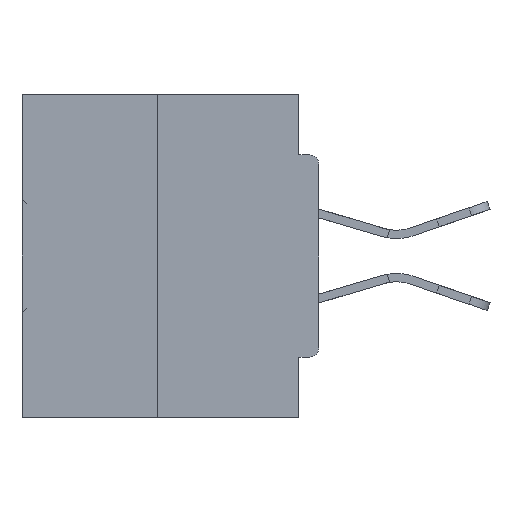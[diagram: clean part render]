
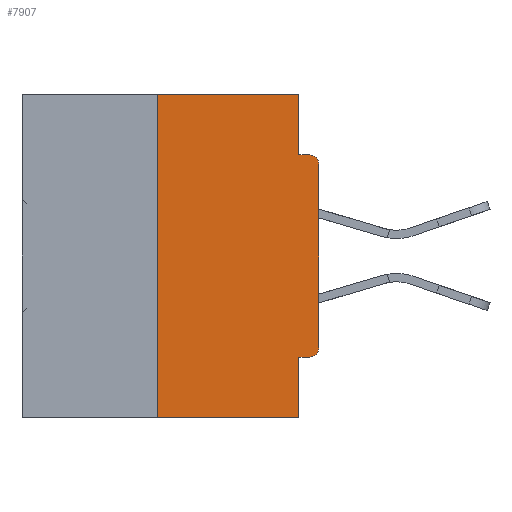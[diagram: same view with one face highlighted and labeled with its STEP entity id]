
A CAD part, left-side view. The second image highlights one B-rep face of the part: STEP entity #7907.
In plain terms, the highlighted planar face has unit normal (-1, 0, 0).
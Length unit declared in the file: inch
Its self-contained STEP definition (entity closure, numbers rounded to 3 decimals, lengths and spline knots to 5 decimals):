
#68 = EDGE_CURVE ( 'NONE', #37832, #5173, #34704, .T. ) ;
#842 = AXIS2_PLACEMENT_3D ( 'NONE', #13772, #17522, #3636 ) ;
#2260 = ORIENTED_EDGE ( 'NONE', *, *, #18033, .F. ) ;
#2802 = CIRCLE ( 'NONE', #25393, 0.015 ) ;
#2816 = CARTESIAN_POINT ( 'NONE',  ( 0., 0.46, -0.5 ) ) ;
#3636 = DIRECTION ( 'NONE',  ( 0., 0., -1. ) ) ;
#4621 = ORIENTED_EDGE ( 'NONE', *, *, #36298, .F. ) ;
#5173 = VERTEX_POINT ( 'NONE', #24727 ) ;
#6350 = VERTEX_POINT ( 'NONE', #41463 ) ;
#7907 = ADVANCED_FACE ( 'NONE', ( #33130 ), #37365, .F. ) ;
#7969 = VECTOR ( 'NONE', #12500, 39.37008 ) ;
#8008 = AXIS2_PLACEMENT_3D ( 'NONE', #12619, #29827, #40417 ) ;
#8057 = CARTESIAN_POINT ( 'NONE',  ( 0., 0.015, -0.4065 ) ) ;
#8179 = VERTEX_POINT ( 'NONE', #10963 ) ;
#8391 = CARTESIAN_POINT ( 'NONE',  ( 0., 0.015, -0.3915 ) ) ;
#8862 = EDGE_CURVE ( 'NONE', #6350, #8179, #31970, .T. ) ;
#10740 = ORIENTED_EDGE ( 'NONE', *, *, #24959, .T. ) ;
#10963 = CARTESIAN_POINT ( 'NONE',  ( 0., 0.031, 0. ) ) ;
#12485 = CARTESIAN_POINT ( 'NONE',  ( 0., 0.031, -0.5 ) ) ;
#12500 = DIRECTION ( 'NONE',  ( 0., -1., 0. ) ) ;
#12554 = EDGE_CURVE ( 'NONE', #15372, #35656, #46511, .T. ) ;
#12619 = CARTESIAN_POINT ( 'NONE',  ( 0., 0.46, 0. ) ) ;
#13407 = ORIENTED_EDGE ( 'NONE', *, *, #38456, .T. ) ;
#13772 = CARTESIAN_POINT ( 'NONE',  ( 0., 0.015, -0.1085 ) ) ;
#14256 = CARTESIAN_POINT ( 'NONE',  ( 0., 0.031, -0.5 ) ) ;
#15091 = LINE ( 'NONE', #36311, #45833 ) ;
#15372 = VERTEX_POINT ( 'NONE', #19482 ) ;
#15651 = EDGE_LOOP ( 'NONE', ( #20581, #33286, #10740, #20710, #2260, #42839, #32192, #13407, #17496, #4621 ) ) ;
#17496 = ORIENTED_EDGE ( 'NONE', *, *, #28105, .F. ) ;
#17522 = DIRECTION ( 'NONE',  ( -1., 0., 0. ) ) ;
#18033 = EDGE_CURVE ( 'NONE', #22012, #15372, #15091, .T. ) ;
#19200 = DIRECTION ( 'NONE',  ( 0., 0., -1. ) ) ;
#19482 = CARTESIAN_POINT ( 'NONE',  ( 0., 0.031, -0.4065 ) ) ;
#19900 = VERTEX_POINT ( 'NONE', #40182 ) ;
#20055 = VERTEX_POINT ( 'NONE', #34281 ) ;
#20581 = ORIENTED_EDGE ( 'NONE', *, *, #8862, .F. ) ;
#20710 = ORIENTED_EDGE ( 'NONE', *, *, #12554, .F. ) ;
#22012 = VERTEX_POINT ( 'NONE', #8057 ) ;
#22480 = DIRECTION ( 'NONE',  ( 0., -1., 0. ) ) ;
#23924 = EDGE_CURVE ( 'NONE', #22012, #37832, #2802, .T. ) ;
#24554 = VECTOR ( 'NONE', #38696, 39.37008 ) ;
#24727 = CARTESIAN_POINT ( 'NONE',  ( 0., 0., -0.1085 ) ) ;
#24959 = EDGE_CURVE ( 'NONE', #19900, #35656, #35084, .T. ) ;
#25393 = AXIS2_PLACEMENT_3D ( 'NONE', #8391, #33586, #44413 ) ;
#25559 = CARTESIAN_POINT ( 'NONE',  ( 0., 0.031, -0.0935 ) ) ;
#25653 = CIRCLE ( 'NONE', #842, 0.015 ) ;
#25705 = CARTESIAN_POINT ( 'NONE',  ( 0., 0., -0.3915 ) ) ;
#26030 = CARTESIAN_POINT ( 'NONE',  ( 0., 0., -0.0935 ) ) ;
#26274 = LINE ( 'NONE', #40622, #33050 ) ;
#26951 = CARTESIAN_POINT ( 'NONE',  ( 0., 0., 0. ) ) ;
#27694 = VECTOR ( 'NONE', #31538, 39.37008 ) ;
#28058 = VERTEX_POINT ( 'NONE', #25559 ) ;
#28105 = EDGE_CURVE ( 'NONE', #28058, #20055, #29544, .T. ) ;
#28616 = DIRECTION ( 'NONE',  ( 0., 0., -1. ) ) ;
#29544 = LINE ( 'NONE', #26030, #43735 ) ;
#29827 = DIRECTION ( 'NONE',  ( 1., 0., 0. ) ) ;
#31538 = DIRECTION ( 'NONE',  ( 0., -1., 0. ) ) ;
#31970 = LINE ( 'NONE', #46102, #7969 ) ;
#32184 = EDGE_CURVE ( 'NONE', #19900, #6350, #34268, .T. ) ;
#32192 = ORIENTED_EDGE ( 'NONE', *, *, #68, .T. ) ;
#33050 = VECTOR ( 'NONE', #19200, 39.37008 ) ;
#33130 = FACE_OUTER_BOUND ( 'NONE', #15651, .T. ) ;
#33286 = ORIENTED_EDGE ( 'NONE', *, *, #32184, .F. ) ;
#33376 = VECTOR ( 'NONE', #38024, 39.37008 ) ;
#33586 = DIRECTION ( 'NONE',  ( -1., 0., 0. ) ) ;
#34268 = LINE ( 'NONE', #37339, #33376 ) ;
#34281 = CARTESIAN_POINT ( 'NONE',  ( 0., 0.015, -0.0935 ) ) ;
#34704 = LINE ( 'NONE', #26951, #24554 ) ;
#35084 = LINE ( 'NONE', #2816, #27694 ) ;
#35608 = DIRECTION ( 'NONE',  ( 0., 1., 0. ) ) ;
#35656 = VERTEX_POINT ( 'NONE', #12485 ) ;
#36298 = EDGE_CURVE ( 'NONE', #8179, #28058, #26274, .T. ) ;
#36311 = CARTESIAN_POINT ( 'NONE',  ( 0., 0., -0.4065 ) ) ;
#36335 = VECTOR ( 'NONE', #28616, 39.37008 ) ;
#37339 = CARTESIAN_POINT ( 'NONE',  ( 0., 0.25, 0. ) ) ;
#37365 = PLANE ( 'NONE',  #8008 ) ;
#37832 = VERTEX_POINT ( 'NONE', #25705 ) ;
#38024 = DIRECTION ( 'NONE',  ( 0., 0., 1. ) ) ;
#38456 = EDGE_CURVE ( 'NONE', #5173, #20055, #25653, .T. ) ;
#38696 = DIRECTION ( 'NONE',  ( 0., 0., 1. ) ) ;
#40182 = CARTESIAN_POINT ( 'NONE',  ( 0., 0.25, -0.5 ) ) ;
#40417 = DIRECTION ( 'NONE',  ( 0., 0., -1. ) ) ;
#40622 = CARTESIAN_POINT ( 'NONE',  ( 0., 0.031, 0. ) ) ;
#41463 = CARTESIAN_POINT ( 'NONE',  ( 0., 0.25, 0. ) ) ;
#42839 = ORIENTED_EDGE ( 'NONE', *, *, #23924, .T. ) ;
#43735 = VECTOR ( 'NONE', #22480, 39.37008 ) ;
#44413 = DIRECTION ( 'NONE',  ( 0., 0., -1. ) ) ;
#45833 = VECTOR ( 'NONE', #35608, 39.37008 ) ;
#46102 = CARTESIAN_POINT ( 'NONE',  ( 0., 0.46, 0. ) ) ;
#46511 = LINE ( 'NONE', #14256, #36335 ) ;
